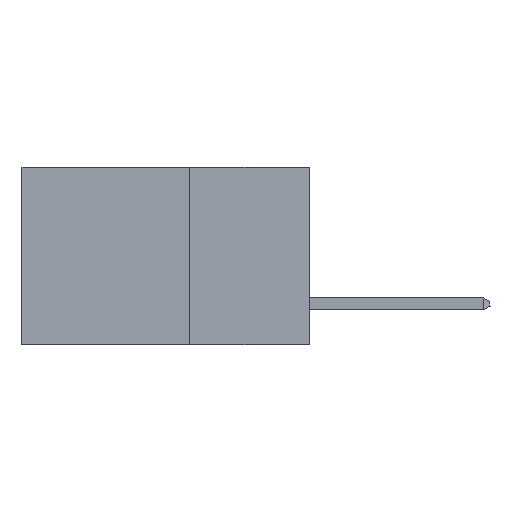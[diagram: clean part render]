
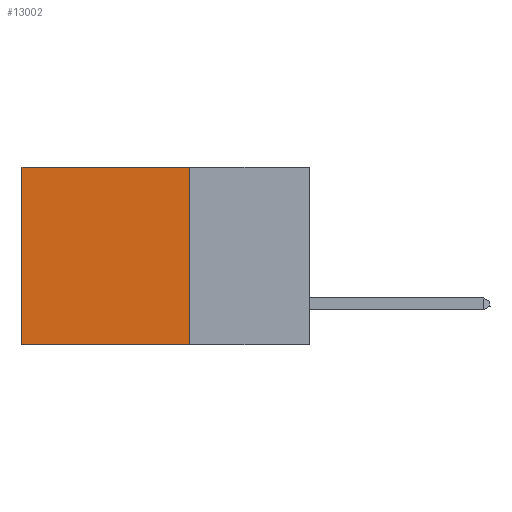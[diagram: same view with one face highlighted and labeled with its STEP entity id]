
A CAD part, left-side view. The second image highlights one B-rep face of the part: STEP entity #13002.
In plain terms, the highlighted planar face has unit normal (-1, 0, 0).
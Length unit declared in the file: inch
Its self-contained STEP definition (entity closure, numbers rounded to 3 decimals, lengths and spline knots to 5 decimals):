
#894 = CARTESIAN_POINT ( 'NONE',  ( 0.2875, 0.25, 0. ) ) ;
#1190 = LINE ( 'NONE', #5760, #1664 ) ;
#1444 = CARTESIAN_POINT ( 'NONE',  ( 0.2875, 0.6, 0. ) ) ;
#1664 = VECTOR ( 'NONE', #10314, 39.37008 ) ;
#1957 = PLANE ( 'NONE',  #11732 ) ;
#2201 = VECTOR ( 'NONE', #5407, 39.37008 ) ;
#2495 = EDGE_CURVE ( 'NONE', #8341, #2557, #6670, .T. ) ;
#2557 = VERTEX_POINT ( 'NONE', #3161 ) ;
#3078 = DIRECTION ( 'NONE',  ( 0., 0., -1. ) ) ;
#3161 = CARTESIAN_POINT ( 'NONE',  ( 0.2875, 0.6, -0.37 ) ) ;
#3324 = LINE ( 'NONE', #12489, #14134 ) ;
#3657 = VERTEX_POINT ( 'NONE', #4216 ) ;
#4216 = CARTESIAN_POINT ( 'NONE',  ( 0.2875, 0.25, 0. ) ) ;
#4418 = EDGE_CURVE ( 'NONE', #3657, #9068, #1190, .T. ) ;
#5400 = DIRECTION ( 'NONE',  ( 1., 0., 0. ) ) ;
#5407 = DIRECTION ( 'NONE',  ( 0., 1., 0. ) ) ;
#5760 = CARTESIAN_POINT ( 'NONE',  ( 0.2875, 0.25, 0. ) ) ;
#6338 = ORIENTED_EDGE ( 'NONE', *, *, #4418, .T. ) ;
#6419 = CARTESIAN_POINT ( 'NONE',  ( 0.2875, 0.25, -0.37 ) ) ;
#6633 = DIRECTION ( 'NONE',  ( 0., 0., -1. ) ) ;
#6670 = LINE ( 'NONE', #11132, #2201 ) ;
#6836 = DIRECTION ( 'NONE',  ( 0., 0., -1. ) ) ;
#8121 = ORIENTED_EDGE ( 'NONE', *, *, #2495, .F. ) ;
#8335 = EDGE_CURVE ( 'NONE', #3657, #8341, #13487, .T. ) ;
#8341 = VERTEX_POINT ( 'NONE', #6419 ) ;
#8786 = CARTESIAN_POINT ( 'NONE',  ( 0.2875, 0.25, 0. ) ) ;
#8977 = ORIENTED_EDGE ( 'NONE', *, *, #8335, .F. ) ;
#9068 = VERTEX_POINT ( 'NONE', #1444 ) ;
#10314 = DIRECTION ( 'NONE',  ( 0., 1., 0. ) ) ;
#10408 = ORIENTED_EDGE ( 'NONE', *, *, #13748, .T. ) ;
#11132 = CARTESIAN_POINT ( 'NONE',  ( 0.2875, 0.25, -0.37 ) ) ;
#11363 = VECTOR ( 'NONE', #6633, 39.37008 ) ;
#11471 = EDGE_LOOP ( 'NONE', ( #10408, #8121, #8977, #6338 ) ) ;
#11732 = AXIS2_PLACEMENT_3D ( 'NONE', #894, #5400, #3078 ) ;
#12031 = FACE_OUTER_BOUND ( 'NONE', #11471, .T. ) ;
#12489 = CARTESIAN_POINT ( 'NONE',  ( 0.2875, 0.6, 0. ) ) ;
#13002 = ADVANCED_FACE ( 'NONE', ( #12031 ), #1957, .F. ) ;
#13487 = LINE ( 'NONE', #8786, #11363 ) ;
#13748 = EDGE_CURVE ( 'NONE', #9068, #2557, #3324, .T. ) ;
#14134 = VECTOR ( 'NONE', #6836, 39.37008 ) ;
